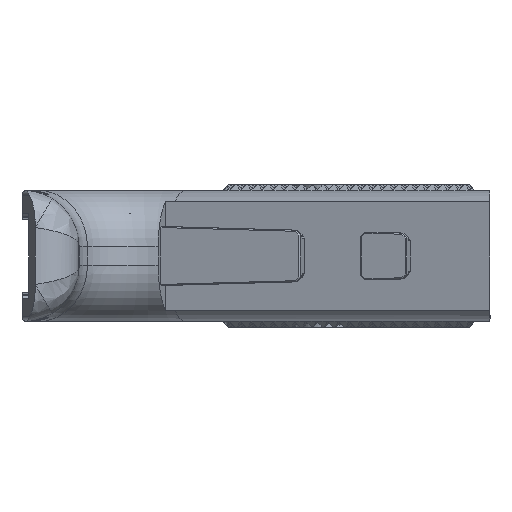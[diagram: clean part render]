
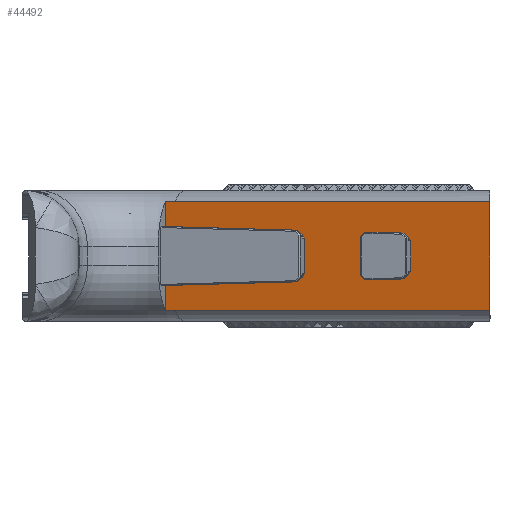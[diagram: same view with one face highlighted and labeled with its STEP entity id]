
A CAD part, left-side view. The second image highlights one B-rep face of the part: STEP entity #44492.
In plain terms, the highlighted planar face has unit normal (-0.951, 0.309, 0).
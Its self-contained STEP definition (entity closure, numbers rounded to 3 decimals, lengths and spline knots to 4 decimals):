
#634=FACE_BOUND('',#8641,.T.);
#3020=PLANE('',#47364);
#5739=FACE_OUTER_BOUND('',#8640,.T.);
#8640=EDGE_LOOP('',(#39702,#39703,#39704,#39705,#39706,#39707,#39708,#39709,
#39710,#39711,#39712,#39713));
#8641=EDGE_LOOP('',(#39714,#39715,#39716,#39717,#39718,#39719,#39720,#39721,
#39722));
#13714=LINE('',#84866,#19124);
#13732=LINE('',#84904,#19142);
#13740=LINE('',#84921,#19150);
#13745=LINE('',#84930,#19155);
#13747=LINE('',#84933,#19157);
#13749=LINE('',#84938,#19159);
#13751=LINE('',#84942,#19161);
#13753=LINE('',#84945,#19163);
#13755=LINE('',#84949,#19165);
#13756=LINE('',#84951,#19166);
#13762=LINE('',#84964,#19172);
#13764=LINE('',#84968,#19174);
#13765=LINE('',#84971,#19175);
#13767=LINE('',#84975,#19177);
#13768=LINE('',#84985,#19178);
#13769=LINE('',#84987,#19179);
#13770=LINE('',#84989,#19180);
#13771=LINE('',#84999,#19181);
#13772=LINE('',#85000,#19182);
#19124=VECTOR('',#57477,0.3937);
#19142=VECTOR('',#57513,0.3937);
#19150=VECTOR('',#57527,0.3937);
#19155=VECTOR('',#57536,0.3937);
#19157=VECTOR('',#57540,0.3937);
#19159=VECTOR('',#57544,0.3937);
#19161=VECTOR('',#57548,0.3937);
#19163=VECTOR('',#57552,0.3937);
#19165=VECTOR('',#57556,0.3937);
#19166=VECTOR('',#57559,0.3937);
#19172=VECTOR('',#57575,0.3937);
#19174=VECTOR('',#57579,0.3937);
#19175=VECTOR('',#57582,0.3937);
#19177=VECTOR('',#57586,0.3937);
#19178=VECTOR('',#57587,0.3937);
#19179=VECTOR('',#57588,0.3937);
#19180=VECTOR('',#57589,0.3937);
#19181=VECTOR('',#57590,0.3937);
#19182=VECTOR('',#57591,0.3937);
#20197=B_SPLINE_CURVE_WITH_KNOTS('',3,(#84977,#84978,#84979,#84980,#84981,
#84982,#84983),.UNSPECIFIED.,.F.,.F.,(4,3,4),(0.,0.1181,0.2155),
 .UNSPECIFIED.);
#20198=B_SPLINE_CURVE_WITH_KNOTS('',3,(#84991,#84992,#84993,#84994,#84995,
#84996,#84997),.UNSPECIFIED.,.F.,.F.,(4,3,4),(-0.2155,-0.1181,
0.),.UNSPECIFIED.);
#22867=VERTEX_POINT('',#84863);
#22868=VERTEX_POINT('',#84865);
#22878=VERTEX_POINT('',#84901);
#22879=VERTEX_POINT('',#84903);
#22884=VERTEX_POINT('',#84918);
#22885=VERTEX_POINT('',#84920);
#22887=VERTEX_POINT('',#84929);
#22888=VERTEX_POINT('',#84935);
#22889=VERTEX_POINT('',#84937);
#22890=VERTEX_POINT('',#84941);
#22891=VERTEX_POINT('',#84947);
#22893=VERTEX_POINT('',#84962);
#22894=VERTEX_POINT('',#84966);
#22895=VERTEX_POINT('',#84970);
#22896=VERTEX_POINT('',#84974);
#22897=VERTEX_POINT('',#84976);
#22898=VERTEX_POINT('',#84984);
#22899=VERTEX_POINT('',#84986);
#22900=VERTEX_POINT('',#84988);
#22901=VERTEX_POINT('',#84990);
#22902=VERTEX_POINT('',#84998);
#28589=EDGE_CURVE('',#22868,#22867,#13714,.T.);
#28607=EDGE_CURVE('',#22878,#22879,#13732,.T.);
#28615=EDGE_CURVE('',#22884,#22885,#13740,.F.);
#28620=EDGE_CURVE('',#22868,#22887,#13745,.F.);
#28622=EDGE_CURVE('',#22884,#22887,#13747,.T.);
#28624=EDGE_CURVE('',#22888,#22889,#13749,.F.);
#28626=EDGE_CURVE('',#22890,#22889,#13751,.T.);
#28628=EDGE_CURVE('',#22888,#22885,#13753,.T.);
#28630=EDGE_CURVE('',#22891,#22867,#13755,.F.);
#28631=EDGE_CURVE('',#22890,#22891,#13756,.F.);
#28637=EDGE_CURVE('',#22893,#22878,#13762,.F.);
#28639=EDGE_CURVE('',#22893,#22894,#13764,.T.);
#28640=EDGE_CURVE('',#22879,#22895,#13765,.F.);
#28642=EDGE_CURVE('',#22896,#22894,#13767,.T.);
#28643=EDGE_CURVE('',#22897,#22896,#20197,.T.);
#28644=EDGE_CURVE('',#22898,#22897,#13768,.T.);
#28645=EDGE_CURVE('',#22899,#22898,#13769,.T.);
#28646=EDGE_CURVE('',#22900,#22899,#13770,.T.);
#28647=EDGE_CURVE('',#22901,#22900,#20198,.T.);
#28648=EDGE_CURVE('',#22902,#22901,#13771,.T.);
#28649=EDGE_CURVE('',#22902,#22895,#13772,.T.);
#39702=ORIENTED_EDGE('',*,*,#28639,.T.);
#39703=ORIENTED_EDGE('',*,*,#28642,.F.);
#39704=ORIENTED_EDGE('',*,*,#28643,.F.);
#39705=ORIENTED_EDGE('',*,*,#28644,.F.);
#39706=ORIENTED_EDGE('',*,*,#28645,.F.);
#39707=ORIENTED_EDGE('',*,*,#28646,.F.);
#39708=ORIENTED_EDGE('',*,*,#28647,.F.);
#39709=ORIENTED_EDGE('',*,*,#28648,.F.);
#39710=ORIENTED_EDGE('',*,*,#28649,.T.);
#39711=ORIENTED_EDGE('',*,*,#28640,.F.);
#39712=ORIENTED_EDGE('',*,*,#28607,.F.);
#39713=ORIENTED_EDGE('',*,*,#28637,.F.);
#39714=ORIENTED_EDGE('',*,*,#28589,.T.);
#39715=ORIENTED_EDGE('',*,*,#28630,.F.);
#39716=ORIENTED_EDGE('',*,*,#28631,.F.);
#39717=ORIENTED_EDGE('',*,*,#28626,.T.);
#39718=ORIENTED_EDGE('',*,*,#28624,.F.);
#39719=ORIENTED_EDGE('',*,*,#28628,.T.);
#39720=ORIENTED_EDGE('',*,*,#28615,.F.);
#39721=ORIENTED_EDGE('',*,*,#28622,.T.);
#39722=ORIENTED_EDGE('',*,*,#28620,.F.);
#44492=ADVANCED_FACE('',(#5739,#634),#3020,.T.);
#47364=AXIS2_PLACEMENT_3D('',#84973,#57584,#57585);
#57477=DIRECTION('',(0.,0.,1.));
#57513=DIRECTION('',(0.,0.,1.));
#57527=DIRECTION('',(0.216,0.664,-0.716));
#57536=DIRECTION('',(0.221,0.681,0.698));
#57540=DIRECTION('',(0.309,0.951,-0.026));
#57544=DIRECTION('',(-0.216,-0.664,-0.716));
#57548=DIRECTION('',(-0.309,-0.951,-0.026));
#57552=DIRECTION('',(0.,0.,-1.));
#57556=DIRECTION('',(-0.12,-0.37,0.921));
#57559=DIRECTION('',(-0.221,-0.681,0.698));
#57575=DIRECTION('',(0.216,0.664,-0.716));
#57579=DIRECTION('',(0.309,0.951,-0.026));
#57582=DIRECTION('',(-0.216,-0.664,-0.716));
#57584=DIRECTION('center_axis',(-0.951,0.309,0.));
#57585=DIRECTION('ref_axis',(0.,0.,
1.));
#57586=DIRECTION('',(0.,0.,1.));
#57587=DIRECTION('',(0.309,0.951,0.));
#57588=DIRECTION('',(0.,0.,-1.));
#57589=DIRECTION('',(-0.309,-0.951,0.));
#57590=DIRECTION('',(0.,0.,1.));
#57591=DIRECTION('',(-0.309,-0.951,-0.026));
#84863=CARTESIAN_POINT('',(-2.8962,-0.8838,-0.6352));
#84865=CARTESIAN_POINT('',(-2.8962,-0.8838,-0.9101));
#84866=CARTESIAN_POINT('',(-2.8962,-0.8838,-0.7677));
#84901=CARTESIAN_POINT('',(-2.7262,-0.3607,-0.9245));
#84903=CARTESIAN_POINT('',(-2.7262,-0.3607,-0.6109));
#84904=CARTESIAN_POINT('',(-2.7262,-0.3607,-0.9154));
#84918=CARTESIAN_POINT('',(-3.0247,-1.2792,-0.909));
#84920=CARTESIAN_POINT('',(-3.0277,-1.2886,-0.8989));
#84921=CARTESIAN_POINT('',(-2.9908,-1.1749,-1.0217));
#84929=CARTESIAN_POINT('',(-2.8992,-0.8932,-0.9197));
#84930=CARTESIAN_POINT('',(-2.8709,-0.806,-0.8303));
#84933=CARTESIAN_POINT('',(-3.0469,-1.3476,-0.9072));
#84935=CARTESIAN_POINT('',(-3.0277,-1.2886,-0.6365));
#84937=CARTESIAN_POINT('',(-3.0247,-1.2792,-0.6264));
#84938=CARTESIAN_POINT('',(-2.9908,-1.1749,-0.5138));
#84941=CARTESIAN_POINT('',(-2.8992,-0.8932,-0.6158));
#84942=CARTESIAN_POINT('',(-3.0469,-1.3476,-0.6283));
#84945=CARTESIAN_POINT('',(-3.0277,-1.2886,-0.899));
#84947=CARTESIAN_POINT('',(-2.8984,-0.8905,-0.6185));
#84949=CARTESIAN_POINT('',(-2.885,-0.8493,-0.7213));
#84951=CARTESIAN_POINT('',(-2.8709,-0.806,-0.7051));
#84962=CARTESIAN_POINT('',(-2.7232,-0.3514,-0.9346));
#84964=CARTESIAN_POINT('',(-2.7647,-0.479,-0.7968));
#84966=CARTESIAN_POINT('',(-2.3324,0.8513,-0.9677));
#84968=CARTESIAN_POINT('',(-3.0469,-1.3476,-0.9072));
#84970=CARTESIAN_POINT('',(-2.7232,-0.3514,-0.6008));
#84971=CARTESIAN_POINT('',(-2.7647,-0.479,-0.7386));
#84973=CARTESIAN_POINT('Origin',(-2.8375,-0.7031,-0.7677));
#84974=CARTESIAN_POINT('',(-2.3324,0.8513,-1.2459));
#84975=CARTESIAN_POINT('',(-2.3324,0.8513,-1.0302));
#84976=CARTESIAN_POINT('',(-2.3592,0.7689,-1.2425));
#84977=CARTESIAN_POINT('Ctrl Pts',(-2.3592,0.7689,
-1.2425));
#84978=CARTESIAN_POINT('Ctrl Pts',(-2.3544,0.7836,
-1.2425));
#84979=CARTESIAN_POINT('Ctrl Pts',(-2.3495,0.7986,
-1.2428));
#84980=CARTESIAN_POINT('Ctrl Pts',(-2.3446,0.8138,
-1.2435));
#84981=CARTESIAN_POINT('Ctrl Pts',(-2.3405,0.8264,
-1.2441));
#84982=CARTESIAN_POINT('Ctrl Pts',(-2.3365,0.8388,
-1.2449));
#84983=CARTESIAN_POINT('Ctrl Pts',(-2.3324,0.8513,-1.2459));
#84984=CARTESIAN_POINT('',(-3.2516,-1.9775,-1.2425));
#84985=CARTESIAN_POINT('',(-2.1969,1.2684,-1.2425));
#84986=CARTESIAN_POINT('',(-3.2516,-1.9775,-0.2929));
#84987=CARTESIAN_POINT('',(-3.2516,-1.9775,-0.3839));
#84988=CARTESIAN_POINT('',(-2.3592,0.7689,-0.2929));
#84989=CARTESIAN_POINT('',(-2.6906,-0.2509,-0.2929));
#84990=CARTESIAN_POINT('',(-2.3324,0.8513,-0.2895));
#84991=CARTESIAN_POINT('Ctrl Pts',(-2.3324,0.8513,-0.2895));
#84992=CARTESIAN_POINT('Ctrl Pts',(-2.3365,0.8388,
-0.2905));
#84993=CARTESIAN_POINT('Ctrl Pts',(-2.3405,0.8264,
-0.2913));
#84994=CARTESIAN_POINT('Ctrl Pts',(-2.3446,0.8138,
-0.2919));
#84995=CARTESIAN_POINT('Ctrl Pts',(-2.3495,0.7986,
-0.2926));
#84996=CARTESIAN_POINT('Ctrl Pts',(-2.3544,0.7836,
-0.2929));
#84997=CARTESIAN_POINT('Ctrl Pts',(-2.3592,0.7689,
-0.2929));
#84998=CARTESIAN_POINT('',(-2.3324,0.8513,-0.5677));
#84999=CARTESIAN_POINT('',(-2.3324,0.8513,-0.7677));
#85000=CARTESIAN_POINT('',(-3.0469,-1.3476,-0.6283));
